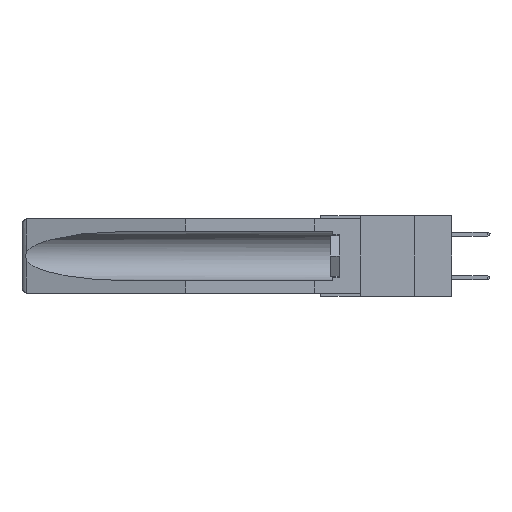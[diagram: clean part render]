
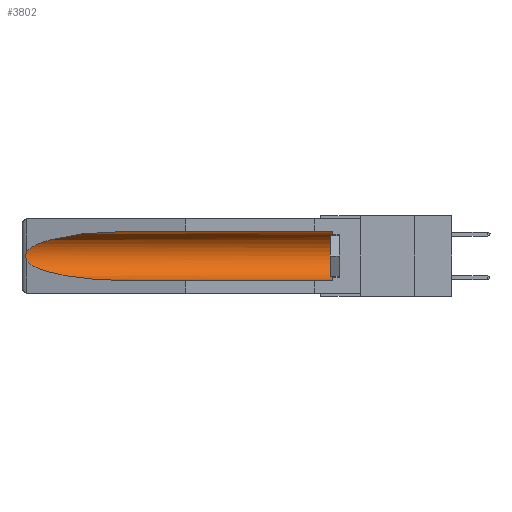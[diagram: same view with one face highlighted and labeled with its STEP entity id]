
A CAD part, left-side view. The second image highlights one B-rep face of the part: STEP entity #3802.
In plain terms, the highlighted cylindrical face has radius 2.857 mm (diameter 5.715 mm), a partial arc.
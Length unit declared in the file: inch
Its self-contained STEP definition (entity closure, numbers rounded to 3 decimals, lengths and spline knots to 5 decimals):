
#25 = VERTEX_POINT ( 'NONE', #2825 ) ;
#371 = EDGE_CURVE ( 'NONE', #25, #4860, #7858, .T. ) ;
#409 = VECTOR ( 'NONE', #7319, 39.37008 ) ;
#466 = CARTESIAN_POINT ( 'NONE',  ( 0.26537, 1.52718, -0.19328 ) ) ;
#1154 = DIRECTION ( 'NONE',  ( 0., 0., 1. ) ) ;
#1640 = CARTESIAN_POINT ( 'NONE',  ( 0.155, 1.07973, -0.284 ) ) ;
#2045 = VERTEX_POINT ( 'NONE', #10842 ) ;
#2055 = EDGE_CURVE ( 'NONE', #2173, #25, #16476, .T. ) ;
#2173 = VERTEX_POINT ( 'NONE', #2410 ) ;
#2410 = CARTESIAN_POINT ( 'NONE',  ( 0.155, 0.126, -0.284 ) ) ;
#2712 = CARTESIAN_POINT ( 'NONE',  ( 0.155, -0.30754, -0.284 ) ) ;
#2825 = CARTESIAN_POINT ( 'NONE',  ( 0.155, 0.126, -0.059 ) ) ;
#3034 = CARTESIAN_POINT ( 'NONE',  ( 0.155, 0.126, -0.1715 ) ) ;
#3058 = CARTESIAN_POINT ( 'NONE',  ( 0.26655, 1.53094, -0.18657 ) ) ;
#3187 = CARTESIAN_POINT ( 'NONE',  ( 0.25451, 1.48313, -0.09465 ) ) ;
#3439 = ORIENTED_EDGE ( 'NONE', *, *, #2055, .T. ) ;
#3802 = ADVANCED_FACE ( 'NONE', ( #6275 ), #12433, .F. ) ;
#4549 = LINE ( 'NONE', #2712, #15937 ) ;
#4860 = VERTEX_POINT ( 'NONE', #8248 ) ;
#5060 = DIRECTION ( 'NONE',  ( 0., 1., 0. ) ) ;
#5547 = CARTESIAN_POINT ( 'NONE',  ( 0.26654, 1.53092, -0.15636 ) ) ;
#5625 = ORIENTED_EDGE ( 'NONE', *, *, #9627, .F. ) ;
#5661 = CARTESIAN_POINT ( 'NONE',  ( 0.26537, 1.52718, -0.14972 ) ) ;
#6130 = CARTESIAN_POINT ( 'NONE',  ( 0.155, 1.07973, -0.059 ) ) ;
#6194 = CARTESIAN_POINT ( 'NONE',  ( 0.21114, 1.30732, -0.059 ) ) ;
#6275 = FACE_OUTER_BOUND ( 'NONE', #15684, .T. ) ;
#6363 = CARTESIAN_POINT ( 'NONE',  ( 0.155, -0.30754, -0.1715 ) ) ;
#6484 = AXIS2_PLACEMENT_3D ( 'NONE', #6363, #5060, #1154 ) ;
#6963 =( BOUNDED_CURVE ( )  B_SPLINE_CURVE ( 3, ( #466, #10646, #10533, #1640 ),
 .UNSPECIFIED., .F., .F. ) 
 B_SPLINE_CURVE_WITH_KNOTS ( ( 4, 4 ),
 ( 0.1948, 1.5708 ),
 .UNSPECIFIED. ) 
 CURVE ( )  GEOMETRIC_REPRESENTATION_ITEM ( )  RATIONAL_B_SPLINE_CURVE ( ( 1., 0.848, 0.848, 1. ) ) 
 REPRESENTATION_ITEM ( '' )  );
#7319 = DIRECTION ( 'NONE',  ( 0., 1., 0. ) ) ;
#7503 = CARTESIAN_POINT ( 'NONE',  ( 0.155, -0.30754, -0.059 ) ) ;
#7858 = LINE ( 'NONE', #7503, #409 ) ;
#8185 = CARTESIAN_POINT ( 'NONE',  ( 0.2673, 1.53269, -0.17917 ) ) ;
#8248 = CARTESIAN_POINT ( 'NONE',  ( 0.155, 1.07973, -0.059 ) ) ;
#8671 = EDGE_CURVE ( 'NONE', #11415, #2045, #6963, .T. ) ;
#9627 = EDGE_CURVE ( 'NONE', #2173, #2045, #4549, .T. ) ;
#9738 = DIRECTION ( 'NONE',  ( 0., 0., 1. ) ) ;
#9918 = EDGE_CURVE ( 'NONE', #13650, #11415, #10812, .T. ) ;
#10334 =( BOUNDED_CURVE ( )  B_SPLINE_CURVE ( 3, ( #6130, #6194, #3187, #15049 ),
 .UNSPECIFIED., .F., .F. ) 
 B_SPLINE_CURVE_WITH_KNOTS ( ( 4, 4 ),
 ( 4.71239, 6.08839 ),
 .UNSPECIFIED. ) 
 CURVE ( )  GEOMETRIC_REPRESENTATION_ITEM ( )  RATIONAL_B_SPLINE_CURVE ( ( 1., 0.848, 0.848, 1. ) ) 
 REPRESENTATION_ITEM ( '' )  );
#10533 = CARTESIAN_POINT ( 'NONE',  ( 0.21114, 1.30732, -0.284 ) ) ;
#10646 = CARTESIAN_POINT ( 'NONE',  ( 0.25451, 1.48313, -0.24835 ) ) ;
#10725 = ORIENTED_EDGE ( 'NONE', *, *, #14876, .T. ) ;
#10812 = B_SPLINE_CURVE_WITH_KNOTS ( 'NONE', 3,
 ( #5661, #15759, #5547, #15808, #13382, #13323, #8185, #3058, #12084, #14596 ),
 .UNSPECIFIED., .F., .F.,
 ( 4, 2, 2, 2, 4 ),
 ( 0., 0.00029, 0.00058, 0.00087, 0.00117 ),
 .UNSPECIFIED. ) ;
#10842 = CARTESIAN_POINT ( 'NONE',  ( 0.155, 1.07973, -0.284 ) ) ;
#11378 = ORIENTED_EDGE ( 'NONE', *, *, #8671, .T. ) ;
#11415 = VERTEX_POINT ( 'NONE', #14928 ) ;
#11597 = ORIENTED_EDGE ( 'NONE', *, *, #371, .T. ) ;
#12006 = AXIS2_PLACEMENT_3D ( 'NONE', #3034, #16002, #9738 ) ;
#12084 = CARTESIAN_POINT ( 'NONE',  ( 0.26597, 1.5296, -0.19026 ) ) ;
#12433 = CYLINDRICAL_SURFACE ( 'NONE', #6484, 0.1125 ) ;
#12440 = ORIENTED_EDGE ( 'NONE', *, *, #9918, .T. ) ;
#12913 = CARTESIAN_POINT ( 'NONE',  ( 0.26537, 1.52718, -0.14972 ) ) ;
#13323 = CARTESIAN_POINT ( 'NONE',  ( 0.2675, 1.53308, -0.17534 ) ) ;
#13382 = CARTESIAN_POINT ( 'NONE',  ( 0.2675, 1.53308, -0.16763 ) ) ;
#13650 = VERTEX_POINT ( 'NONE', #12913 ) ;
#14596 = CARTESIAN_POINT ( 'NONE',  ( 0.26537, 1.52718, -0.19328 ) ) ;
#14876 = EDGE_CURVE ( 'NONE', #4860, #13650, #10334, .T. ) ;
#14928 = CARTESIAN_POINT ( 'NONE',  ( 0.26537, 1.52718, -0.19328 ) ) ;
#15049 = CARTESIAN_POINT ( 'NONE',  ( 0.26537, 1.52718, -0.14972 ) ) ;
#15400 = DIRECTION ( 'NONE',  ( 0., 1., 0. ) ) ;
#15684 = EDGE_LOOP ( 'NONE', ( #10725, #12440, #11378, #5625, #3439, #11597 ) ) ;
#15759 = CARTESIAN_POINT ( 'NONE',  ( 0.26597, 1.52961, -0.15275 ) ) ;
#15808 = CARTESIAN_POINT ( 'NONE',  ( 0.2673, 1.5327, -0.16383 ) ) ;
#15937 = VECTOR ( 'NONE', #15400, 39.37008 ) ;
#16002 = DIRECTION ( 'NONE',  ( 0., -1., 0. ) ) ;
#16476 = CIRCLE ( 'NONE', #12006, 0.1125 ) ;
